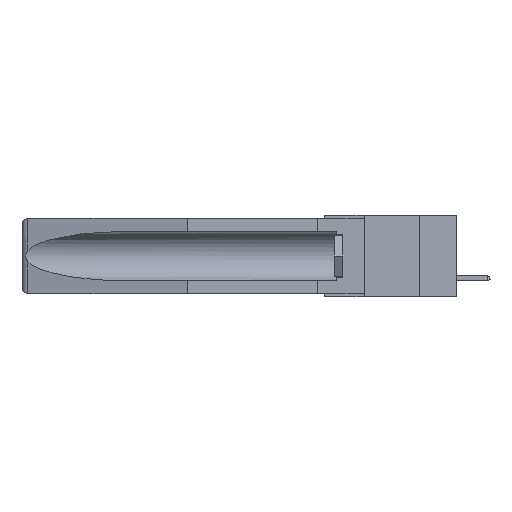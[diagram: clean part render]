
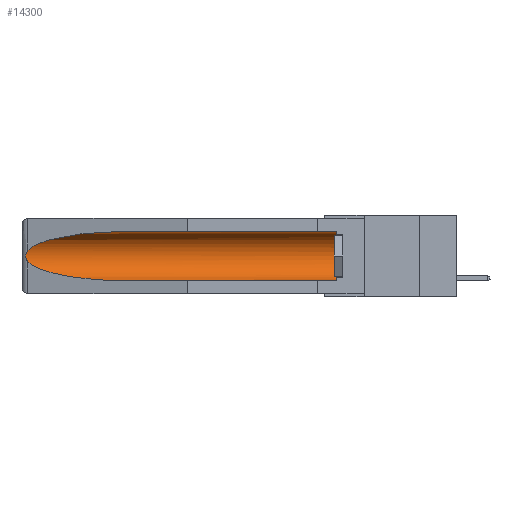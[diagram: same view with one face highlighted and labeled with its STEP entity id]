
A CAD part, left-side view. The second image highlights one B-rep face of the part: STEP entity #14300.
In plain terms, the highlighted cylindrical face has radius 2.857 mm (diameter 5.715 mm), a partial arc.
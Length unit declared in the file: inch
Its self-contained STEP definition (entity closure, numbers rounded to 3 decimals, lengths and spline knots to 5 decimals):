
#966 = CARTESIAN_POINT ( 'NONE',  ( 0.26537, 1.52718, -0.14972 ) ) ;
#1139 = CARTESIAN_POINT ( 'NONE',  ( 0.26537, 1.52718, -0.19328 ) ) ;
#4099 = CARTESIAN_POINT ( 'NONE',  ( 0.155, 1.07973, -0.284 ) ) ;
#4500 = CARTESIAN_POINT ( 'NONE',  ( 0.21114, 1.30732, -0.059 ) ) ;
#4572 = LINE ( 'NONE', #29419, #20969 ) ;
#5084 = CYLINDRICAL_SURFACE ( 'NONE', #13967, 0.1125 ) ;
#5247 = DIRECTION ( 'NONE',  ( 0., 1., 0. ) ) ;
#5250 = DIRECTION ( 'NONE',  ( 0., 1., 0. ) ) ;
#6045 = AXIS2_PLACEMENT_3D ( 'NONE', #13259, #8354, #25088 ) ;
#6058 = CARTESIAN_POINT ( 'NONE',  ( 0.155, 0.126, -0.059 ) ) ;
#6850 = LINE ( 'NONE', #7993, #15086 ) ;
#7186 = EDGE_CURVE ( 'NONE', #18147, #13776, #28103, .T. ) ;
#7304 = CARTESIAN_POINT ( 'NONE',  ( 0.26537, 1.52718, -0.14972 ) ) ;
#7427 = CARTESIAN_POINT ( 'NONE',  ( 0.26654, 1.53092, -0.15636 ) ) ;
#7847 = ORIENTED_EDGE ( 'NONE', *, *, #22923, .T. ) ;
#7993 = CARTESIAN_POINT ( 'NONE',  ( 0.155, -0.30754, -0.284 ) ) ;
#8354 = DIRECTION ( 'NONE',  ( 0., -1., 0. ) ) ;
#8726 = CARTESIAN_POINT ( 'NONE',  ( 0.155, -0.30754, -0.1715 ) ) ;
#8890 = EDGE_CURVE ( 'NONE', #30634, #10708, #18306, .T. ) ;
#9155 = EDGE_CURVE ( 'NONE', #30634, #21705, #6850, .T. ) ;
#9241 = ORIENTED_EDGE ( 'NONE', *, *, #7186, .T. ) ;
#10320 = EDGE_CURVE ( 'NONE', #10708, #10707, #4572, .T. ) ;
#10600 = CARTESIAN_POINT ( 'NONE',  ( 0.2675, 1.53308, -0.17534 ) ) ;
#10707 = VERTEX_POINT ( 'NONE', #13278 ) ;
#10708 = VERTEX_POINT ( 'NONE', #6058 ) ;
#10812 = CARTESIAN_POINT ( 'NONE',  ( 0.26655, 1.53094, -0.18657 ) ) ;
#10830 = ORIENTED_EDGE ( 'NONE', *, *, #10320, .T. ) ;
#11211 = DIRECTION ( 'NONE',  ( 0., 0., 1. ) ) ;
#11791 = CARTESIAN_POINT ( 'NONE',  ( 0.25451, 1.48313, -0.24835 ) ) ;
#12096 = CARTESIAN_POINT ( 'NONE',  ( 0.155, 1.07973, -0.059 ) ) ;
#12124 =( BOUNDED_CURVE ( )  B_SPLINE_CURVE ( 3, ( #12096, #4500, #21160, #14208 ),
 .UNSPECIFIED., .F., .F. ) 
 B_SPLINE_CURVE_WITH_KNOTS ( ( 4, 4 ),
 ( 4.71239, 6.08839 ),
 .UNSPECIFIED. ) 
 CURVE ( )  GEOMETRIC_REPRESENTATION_ITEM ( )  RATIONAL_B_SPLINE_CURVE ( ( 1., 0.848, 0.848, 1. ) ) 
 REPRESENTATION_ITEM ( '' )  );
#12815 = CARTESIAN_POINT ( 'NONE',  ( 0.2673, 1.53269, -0.17917 ) ) ;
#13100 =( BOUNDED_CURVE ( )  B_SPLINE_CURVE ( 3, ( #14410, #11791, #16789, #26034 ),
 .UNSPECIFIED., .F., .F. ) 
 B_SPLINE_CURVE_WITH_KNOTS ( ( 4, 4 ),
 ( 0.1948, 1.5708 ),
 .UNSPECIFIED. ) 
 CURVE ( )  GEOMETRIC_REPRESENTATION_ITEM ( )  RATIONAL_B_SPLINE_CURVE ( ( 1., 0.848, 0.848, 1. ) ) 
 REPRESENTATION_ITEM ( '' )  );
#13259 = CARTESIAN_POINT ( 'NONE',  ( 0.155, 0.126, -0.1715 ) ) ;
#13278 = CARTESIAN_POINT ( 'NONE',  ( 0.155, 1.07973, -0.059 ) ) ;
#13447 = CARTESIAN_POINT ( 'NONE',  ( 0.26537, 1.52718, -0.19328 ) ) ;
#13776 = VERTEX_POINT ( 'NONE', #13447 ) ;
#13967 = AXIS2_PLACEMENT_3D ( 'NONE', #8726, #20780, #11211 ) ;
#14208 = CARTESIAN_POINT ( 'NONE',  ( 0.26537, 1.52718, -0.14972 ) ) ;
#14300 = ADVANCED_FACE ( 'NONE', ( #15125 ), #5084, .F. ) ;
#14367 = ORIENTED_EDGE ( 'NONE', *, *, #9155, .F. ) ;
#14410 = CARTESIAN_POINT ( 'NONE',  ( 0.26537, 1.52718, -0.19328 ) ) ;
#15086 = VECTOR ( 'NONE', #5250, 39.37008 ) ;
#15125 = FACE_OUTER_BOUND ( 'NONE', #16812, .T. ) ;
#16789 = CARTESIAN_POINT ( 'NONE',  ( 0.21114, 1.30732, -0.284 ) ) ;
#16812 = EDGE_LOOP ( 'NONE', ( #7847, #9241, #19364, #14367, #19674, #10830 ) ) ;
#17872 = CARTESIAN_POINT ( 'NONE',  ( 0.26597, 1.5296, -0.19026 ) ) ;
#18147 = VERTEX_POINT ( 'NONE', #966 ) ;
#18306 = CIRCLE ( 'NONE', #6045, 0.1125 ) ;
#19364 = ORIENTED_EDGE ( 'NONE', *, *, #26249, .T. ) ;
#19674 = ORIENTED_EDGE ( 'NONE', *, *, #8890, .T. ) ;
#20160 = CARTESIAN_POINT ( 'NONE',  ( 0.155, 0.126, -0.284 ) ) ;
#20780 = DIRECTION ( 'NONE',  ( 0., 1., 0. ) ) ;
#20969 = VECTOR ( 'NONE', #5247, 39.37008 ) ;
#21160 = CARTESIAN_POINT ( 'NONE',  ( 0.25451, 1.48313, -0.09465 ) ) ;
#21705 = VERTEX_POINT ( 'NONE', #4099 ) ;
#22923 = EDGE_CURVE ( 'NONE', #10707, #18147, #12124, .T. ) ;
#24638 = CARTESIAN_POINT ( 'NONE',  ( 0.2675, 1.53308, -0.16763 ) ) ;
#25088 = DIRECTION ( 'NONE',  ( 0., 0., 1. ) ) ;
#26034 = CARTESIAN_POINT ( 'NONE',  ( 0.155, 1.07973, -0.284 ) ) ;
#26249 = EDGE_CURVE ( 'NONE', #13776, #21705, #13100, .T. ) ;
#27016 = CARTESIAN_POINT ( 'NONE',  ( 0.2673, 1.5327, -0.16383 ) ) ;
#28103 = B_SPLINE_CURVE_WITH_KNOTS ( 'NONE', 3,
 ( #7304, #28705, #7427, #27016, #24638, #10600, #12815, #10812, #17872, #1139 ),
 .UNSPECIFIED., .F., .F.,
 ( 4, 2, 2, 2, 4 ),
 ( 0., 0.00029, 0.00058, 0.00087, 0.00117 ),
 .UNSPECIFIED. ) ;
#28705 = CARTESIAN_POINT ( 'NONE',  ( 0.26597, 1.52961, -0.15275 ) ) ;
#29419 = CARTESIAN_POINT ( 'NONE',  ( 0.155, -0.30754, -0.059 ) ) ;
#30634 = VERTEX_POINT ( 'NONE', #20160 ) ;
